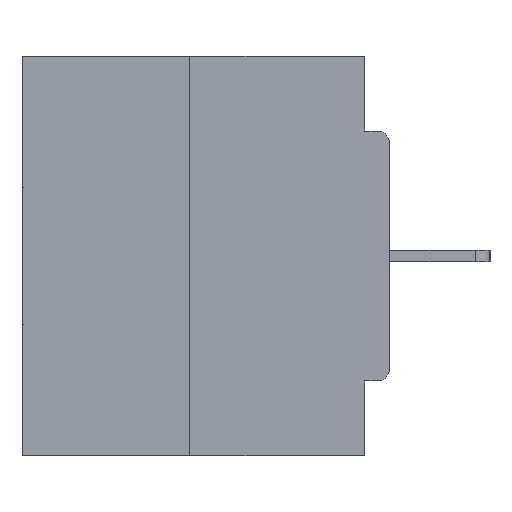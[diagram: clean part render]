
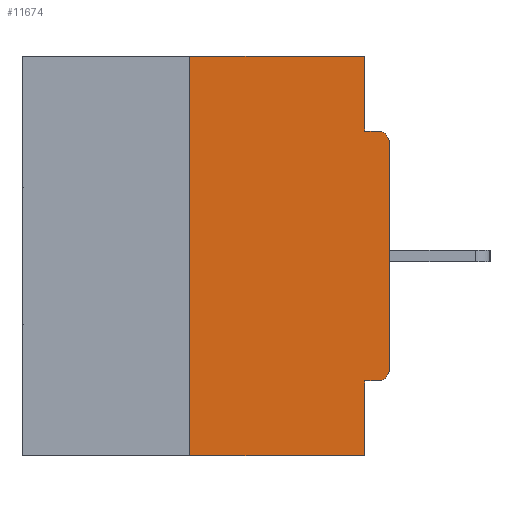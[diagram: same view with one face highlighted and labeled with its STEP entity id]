
A CAD part, left-side view. The second image highlights one B-rep face of the part: STEP entity #11674.
In plain terms, the highlighted planar face has unit normal (-1, 0, 0).
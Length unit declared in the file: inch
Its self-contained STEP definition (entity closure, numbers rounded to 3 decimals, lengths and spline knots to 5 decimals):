
#74 = CARTESIAN_POINT ( 'NONE',  ( 0., 0.015, -0.1085 ) ) ;
#138 = LINE ( 'NONE', #23514, #15460 ) ;
#1010 = EDGE_CURVE ( 'NONE', #16143, #14120, #23718, .T. ) ;
#1432 = LINE ( 'NONE', #22399, #8359 ) ;
#1539 = VERTEX_POINT ( 'NONE', #2810 ) ;
#1920 = VECTOR ( 'NONE', #29428, 39.37008 ) ;
#1969 = CARTESIAN_POINT ( 'NONE',  ( 0., 0.015, -0.3915 ) ) ;
#2362 = ORIENTED_EDGE ( 'NONE', *, *, #21514, .F. ) ;
#2810 = CARTESIAN_POINT ( 'NONE',  ( 0., 0.031, -0.5 ) ) ;
#3288 = CARTESIAN_POINT ( 'NONE',  ( 0., 0.25, 0. ) ) ;
#3727 = VERTEX_POINT ( 'NONE', #32411 ) ;
#3833 = VERTEX_POINT ( 'NONE', #18038 ) ;
#4243 = DIRECTION ( 'NONE',  ( 0., 0., 1. ) ) ;
#4448 = LINE ( 'NONE', #22697, #27540 ) ;
#4480 = ORIENTED_EDGE ( 'NONE', *, *, #28811, .T. ) ;
#4871 = DIRECTION ( 'NONE',  ( 0., 0., -1. ) ) ;
#5910 = CARTESIAN_POINT ( 'NONE',  ( 0., 0.031, -0.0935 ) ) ;
#6246 = VECTOR ( 'NONE', #25686, 39.37008 ) ;
#7103 = LINE ( 'NONE', #12417, #6246 ) ;
#7587 = DIRECTION ( 'NONE',  ( 0., 0., -1. ) ) ;
#7912 = EDGE_CURVE ( 'NONE', #3833, #1539, #15300, .T. ) ;
#7991 = DIRECTION ( 'NONE',  ( 0., 1., 0. ) ) ;
#8359 = VECTOR ( 'NONE', #21733, 39.37008 ) ;
#8875 = AXIS2_PLACEMENT_3D ( 'NONE', #25380, #22804, #12278 ) ;
#10095 = CARTESIAN_POINT ( 'NONE',  ( 0., 0., -0.3915 ) ) ;
#10413 = EDGE_CURVE ( 'NONE', #16933, #11871, #7103, .T. ) ;
#10455 = LINE ( 'NONE', #15792, #11422 ) ;
#10474 = CARTESIAN_POINT ( 'NONE',  ( 0., 0.031, -0.5 ) ) ;
#10549 = EDGE_CURVE ( 'NONE', #11871, #17238, #26528, .T. ) ;
#10575 = ORIENTED_EDGE ( 'NONE', *, *, #7912, .F. ) ;
#10699 = EDGE_CURVE ( 'NONE', #3727, #1539, #1432, .T. ) ;
#11028 = EDGE_CURVE ( 'NONE', #3727, #22461, #23750, .T. ) ;
#11422 = VECTOR ( 'NONE', #23714, 39.37008 ) ;
#11444 = EDGE_CURVE ( 'NONE', #16143, #3833, #138, .T. ) ;
#11674 = ADVANCED_FACE ( 'NONE', ( #17316 ), #27748, .F. ) ;
#11871 = VERTEX_POINT ( 'NONE', #5910 ) ;
#12278 = DIRECTION ( 'NONE',  ( 0., 0., -1. ) ) ;
#12326 = DIRECTION ( 'NONE',  ( 0., 0., 1. ) ) ;
#12417 = CARTESIAN_POINT ( 'NONE',  ( 0., 0.031, 0. ) ) ;
#13257 = ORIENTED_EDGE ( 'NONE', *, *, #10549, .F. ) ;
#13527 = ORIENTED_EDGE ( 'NONE', *, *, #10413, .F. ) ;
#13682 = CARTESIAN_POINT ( 'NONE',  ( 0., 0.015, -0.0935 ) ) ;
#14120 = VERTEX_POINT ( 'NONE', #10095 ) ;
#14543 = EDGE_CURVE ( 'NONE', #25692, #17238, #24753, .T. ) ;
#14901 = CARTESIAN_POINT ( 'NONE',  ( 0., 0.031, 0. ) ) ;
#15137 = DIRECTION ( 'NONE',  ( 0., 0., -1. ) ) ;
#15300 = LINE ( 'NONE', #10474, #32891 ) ;
#15460 = VECTOR ( 'NONE', #7991, 39.37008 ) ;
#15792 = CARTESIAN_POINT ( 'NONE',  ( 0., 0.46, 0. ) ) ;
#15872 = CARTESIAN_POINT ( 'NONE',  ( 0., 0., -0.0935 ) ) ;
#16143 = VERTEX_POINT ( 'NONE', #17433 ) ;
#16933 = VERTEX_POINT ( 'NONE', #14901 ) ;
#17238 = VERTEX_POINT ( 'NONE', #13682 ) ;
#17316 = FACE_OUTER_BOUND ( 'NONE', #21591, .T. ) ;
#17433 = CARTESIAN_POINT ( 'NONE',  ( 0., 0.015, -0.4065 ) ) ;
#17809 = DIRECTION ( 'NONE',  ( -1., 0., 0. ) ) ;
#18038 = CARTESIAN_POINT ( 'NONE',  ( 0., 0.031, -0.4065 ) ) ;
#18969 = ORIENTED_EDGE ( 'NONE', *, *, #10699, .T. ) ;
#20082 = CARTESIAN_POINT ( 'NONE',  ( 0., 0.25, 0. ) ) ;
#20366 = DIRECTION ( 'NONE',  ( -1., 0., 0. ) ) ;
#20554 = ORIENTED_EDGE ( 'NONE', *, *, #11028, .F. ) ;
#21514 = EDGE_CURVE ( 'NONE', #22461, #16933, #10455, .T. ) ;
#21591 = EDGE_LOOP ( 'NONE', ( #2362, #20554, #18969, #10575, #28519, #29968, #4480, #30575, #13257, #13527 ) ) ;
#21733 = DIRECTION ( 'NONE',  ( 0., -1., 0. ) ) ;
#22399 = CARTESIAN_POINT ( 'NONE',  ( 0., 0.46, -0.5 ) ) ;
#22461 = VERTEX_POINT ( 'NONE', #3288 ) ;
#22697 = CARTESIAN_POINT ( 'NONE',  ( 0., 0., 0. ) ) ;
#22804 = DIRECTION ( 'NONE',  ( 1., 0., 0. ) ) ;
#23514 = CARTESIAN_POINT ( 'NONE',  ( 0., 0., -0.4065 ) ) ;
#23714 = DIRECTION ( 'NONE',  ( 0., -1., 0. ) ) ;
#23718 = CIRCLE ( 'NONE', #28084, 0.015 ) ;
#23750 = LINE ( 'NONE', #20082, #28661 ) ;
#23808 = CARTESIAN_POINT ( 'NONE',  ( 0., 0., -0.1085 ) ) ;
#24753 = CIRCLE ( 'NONE', #26379, 0.015 ) ;
#25380 = CARTESIAN_POINT ( 'NONE',  ( 0., 0.46, 0. ) ) ;
#25686 = DIRECTION ( 'NONE',  ( 0., 0., -1. ) ) ;
#25692 = VERTEX_POINT ( 'NONE', #23808 ) ;
#26379 = AXIS2_PLACEMENT_3D ( 'NONE', #74, #17809, #7587 ) ;
#26528 = LINE ( 'NONE', #15872, #1920 ) ;
#27540 = VECTOR ( 'NONE', #12326, 39.37008 ) ;
#27748 = PLANE ( 'NONE',  #8875 ) ;
#28084 = AXIS2_PLACEMENT_3D ( 'NONE', #1969, #20366, #4871 ) ;
#28519 = ORIENTED_EDGE ( 'NONE', *, *, #11444, .F. ) ;
#28661 = VECTOR ( 'NONE', #4243, 39.37008 ) ;
#28811 = EDGE_CURVE ( 'NONE', #14120, #25692, #4448, .T. ) ;
#29428 = DIRECTION ( 'NONE',  ( 0., -1., 0. ) ) ;
#29968 = ORIENTED_EDGE ( 'NONE', *, *, #1010, .T. ) ;
#30575 = ORIENTED_EDGE ( 'NONE', *, *, #14543, .T. ) ;
#32411 = CARTESIAN_POINT ( 'NONE',  ( 0., 0.25, -0.5 ) ) ;
#32891 = VECTOR ( 'NONE', #15137, 39.37008 ) ;
